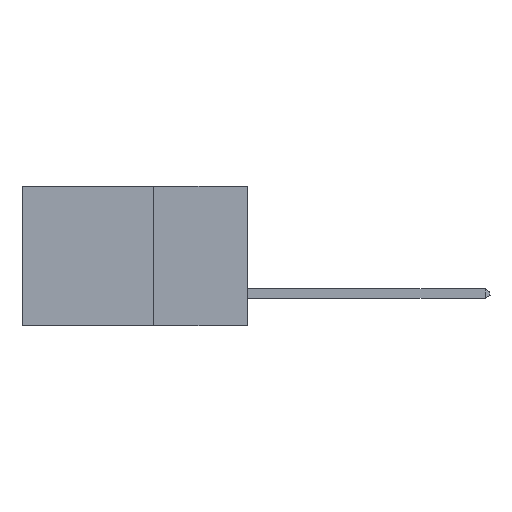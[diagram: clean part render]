
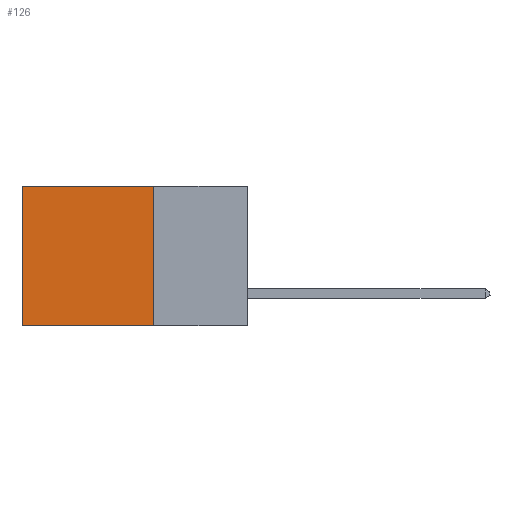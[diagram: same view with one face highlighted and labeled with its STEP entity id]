
A CAD part, left-side view. The second image highlights one B-rep face of the part: STEP entity #126.
In plain terms, the highlighted planar face has unit normal (-1, 0, 0).
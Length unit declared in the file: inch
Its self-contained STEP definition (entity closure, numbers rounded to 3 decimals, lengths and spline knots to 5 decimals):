
#121 = ORIENTED_EDGE ( 'NONE', *, *, #196, .F. ) ;
#126 = ADVANCED_FACE ( 'NONE', ( #3351 ), #5440, .F. ) ;
#196 = EDGE_CURVE ( 'NONE', #4892, #5269, #1504, .T. ) ;
#381 = CARTESIAN_POINT ( 'NONE',  ( 0.298, 0.6, 0. ) ) ;
#584 = VECTOR ( 'NONE', #4666, 39.37008 ) ;
#618 = CARTESIAN_POINT ( 'NONE',  ( 0.298, 0.6, -0.37 ) ) ;
#685 = EDGE_LOOP ( 'NONE', ( #3179, #121, #3658, #2965 ) ) ;
#848 = CARTESIAN_POINT ( 'NONE',  ( 0.298, 0.25, 0. ) ) ;
#1033 = LINE ( 'NONE', #848, #7497 ) ;
#1504 = LINE ( 'NONE', #5436, #584 ) ;
#1632 = CARTESIAN_POINT ( 'NONE',  ( 0.298, 0.25, 0. ) ) ;
#2003 = EDGE_CURVE ( 'NONE', #2559, #5269, #7820, .T. ) ;
#2559 = VERTEX_POINT ( 'NONE', #3570 ) ;
#2965 = ORIENTED_EDGE ( 'NONE', *, *, #9844, .T. ) ;
#2974 = DIRECTION ( 'NONE',  ( 0., 0., -1. ) ) ;
#3051 = VECTOR ( 'NONE', #2974, 39.37008 ) ;
#3179 = ORIENTED_EDGE ( 'NONE', *, *, #2003, .T. ) ;
#3351 = FACE_OUTER_BOUND ( 'NONE', #685, .T. ) ;
#3570 = CARTESIAN_POINT ( 'NONE',  ( 0.298, 0.6, 0. ) ) ;
#3658 = ORIENTED_EDGE ( 'NONE', *, *, #7705, .F. ) ;
#3891 = DIRECTION ( 'NONE',  ( 0., 0., -1. ) ) ;
#3936 = CARTESIAN_POINT ( 'NONE',  ( 0.298, 0.25, -0.37 ) ) ;
#4666 = DIRECTION ( 'NONE',  ( 0., 1., 0. ) ) ;
#4777 = LINE ( 'NONE', #8785, #5983 ) ;
#4892 = VERTEX_POINT ( 'NONE', #3936 ) ;
#5269 = VERTEX_POINT ( 'NONE', #618 ) ;
#5436 = CARTESIAN_POINT ( 'NONE',  ( 0.298, 0.25, -0.37 ) ) ;
#5440 = PLANE ( 'NONE',  #5558 ) ;
#5558 = AXIS2_PLACEMENT_3D ( 'NONE', #9672, #7309, #5912 ) ;
#5904 = DIRECTION ( 'NONE',  ( 0., 1., 0. ) ) ;
#5912 = DIRECTION ( 'NONE',  ( 0., 0., -1. ) ) ;
#5983 = VECTOR ( 'NONE', #3891, 39.37008 ) ;
#7109 = VERTEX_POINT ( 'NONE', #1632 ) ;
#7309 = DIRECTION ( 'NONE',  ( 1., 0., 0. ) ) ;
#7497 = VECTOR ( 'NONE', #5904, 39.37008 ) ;
#7705 = EDGE_CURVE ( 'NONE', #7109, #4892, #4777, .T. ) ;
#7820 = LINE ( 'NONE', #381, #3051 ) ;
#8785 = CARTESIAN_POINT ( 'NONE',  ( 0.298, 0.25, 0. ) ) ;
#9672 = CARTESIAN_POINT ( 'NONE',  ( 0.298, 0.25, 0. ) ) ;
#9844 = EDGE_CURVE ( 'NONE', #7109, #2559, #1033, .T. ) ;
